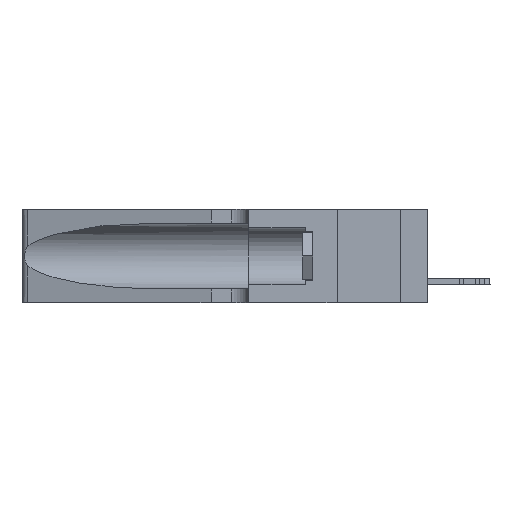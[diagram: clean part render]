
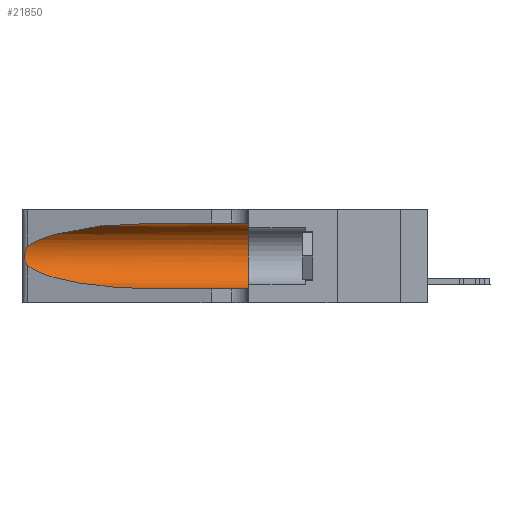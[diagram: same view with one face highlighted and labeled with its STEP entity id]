
A CAD part, left-side view. The second image highlights one B-rep face of the part: STEP entity #21850.
In plain terms, the highlighted cylindrical face has radius 3.308 mm (diameter 6.617 mm), a partial arc.
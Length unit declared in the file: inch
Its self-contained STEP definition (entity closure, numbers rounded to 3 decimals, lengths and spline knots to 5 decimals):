
#223 = FACE_OUTER_BOUND ( 'NONE', #41740, .T. ) ;
#475 = CARTESIAN_POINT ( 'NONE',  ( 0.1305, 0.35, 0.185 ) ) ;
#587 = VERTEX_POINT ( 'NONE', #12736 ) ;
#870 = ORIENTED_EDGE ( 'NONE', *, *, #23243, .T. ) ;
#1257 = CARTESIAN_POINT ( 'NONE',  ( 0.2373, 1.15595, 0.08982 ) ) ;
#1524 = ORIENTED_EDGE ( 'NONE', *, *, #5463, .F. ) ;
#1861 = CARTESIAN_POINT ( 'NONE',  ( 0.25639, 1.23184, 0.21858 ) ) ;
#2933 =( BOUNDED_CURVE ( )  B_SPLINE_CURVE ( 3, ( #22424, #42222, #25912, #22264 ),
 .UNSPECIFIED., .F., .F. ) 
 B_SPLINE_CURVE_WITH_KNOTS ( ( 4, 4 ),
 ( 1.5708, 2.84003 ),
 .UNSPECIFIED. ) 
 CURVE ( )  GEOMETRIC_REPRESENTATION_ITEM ( )  RATIONAL_B_SPLINE_CURVE ( ( 1., 0.87, 0.87, 1. ) ) 
 REPRESENTATION_ITEM ( '' )  );
#5463 = EDGE_CURVE ( 'NONE', #10100, #587, #26725, .T. ) ;
#5940 = DIRECTION ( 'NONE',  ( 0., -1., 0. ) ) ;
#6716 = VECTOR ( 'NONE', #9171, 39.37008 ) ;
#8279 = CIRCLE ( 'NONE', #35297, 0.13025 ) ;
#8772 = CARTESIAN_POINT ( 'NONE',  ( 0.26075, 1.23896, 0.19203 ) ) ;
#9171 = DIRECTION ( 'NONE',  ( 0., -1., 0. ) ) ;
#10028 = VERTEX_POINT ( 'NONE', #22106 ) ;
#10100 = VERTEX_POINT ( 'NONE', #35919 ) ;
#12147 = VERTEX_POINT ( 'NONE', #14419 ) ;
#12736 = CARTESIAN_POINT ( 'NONE',  ( 0.1305, 0.35, 0.31525 ) ) ;
#13600 = ORIENTED_EDGE ( 'NONE', *, *, #14310, .T. ) ;
#14310 = EDGE_CURVE ( 'NONE', #16075, #12147, #15464, .T. ) ;
#14419 = CARTESIAN_POINT ( 'NONE',  ( 0.1305, 0.35, 0.05475 ) ) ;
#14568 = CARTESIAN_POINT ( 'NONE',  ( 0.1305, 1.61858, 0.31525 ) ) ;
#15225 = CARTESIAN_POINT ( 'NONE',  ( 0.25555, 1.22994, 0.2215 ) ) ;
#15379 = CARTESIAN_POINT ( 'NONE',  ( 0.25787, 1.23484, 0.2124 ) ) ;
#15464 = LINE ( 'NONE', #30836, #6716 ) ;
#16075 = VERTEX_POINT ( 'NONE', #19417 ) ;
#17634 = CARTESIAN_POINT ( 'NONE',  ( 0.1305, 1.61858, 0.185 ) ) ;
#17783 = CARTESIAN_POINT ( 'NONE',  ( 0.1305, 0.72297, 0.05475 ) ) ;
#17888 = ORIENTED_EDGE ( 'NONE', *, *, #30081, .T. ) ;
#18008 = VECTOR ( 'NONE', #5940, 39.37008 ) ;
#19417 = CARTESIAN_POINT ( 'NONE',  ( 0.1305, 0.72297, 0.05475 ) ) ;
#21526 = CARTESIAN_POINT ( 'NONE',  ( 0.26075, 1.23896, 0.178 ) ) ;
#21850 = ADVANCED_FACE ( 'NONE', ( #223 ), #28533, .F. ) ;
#21956 = CARTESIAN_POINT ( 'NONE',  ( 0.25854, 1.2359, 0.20912 ) ) ;
#22106 = CARTESIAN_POINT ( 'NONE',  ( 0.25487, 1.22718, 0.14631 ) ) ;
#22264 = CARTESIAN_POINT ( 'NONE',  ( 0.25487, 1.22718, 0.22369 ) ) ;
#22424 = CARTESIAN_POINT ( 'NONE',  ( 0.1305, 0.72297, 0.31525 ) ) ;
#22768 = CARTESIAN_POINT ( 'NONE',  ( 0.25487, 1.22718, 0.22369 ) ) ;
#23243 = EDGE_CURVE ( 'NONE', #10100, #38508, #2933, .T. ) ;
#23575 = DIRECTION ( 'NONE',  ( 0., 1., 0. ) ) ;
#24788 = ORIENTED_EDGE ( 'NONE', *, *, #33444, .T. ) ;
#24831 = CARTESIAN_POINT ( 'NONE',  ( 0.26017, 1.23833, 0.17102 ) ) ;
#24858 = AXIS2_PLACEMENT_3D ( 'NONE', #17634, #40010, #40598 ) ;
#24983 = CARTESIAN_POINT ( 'NONE',  ( 0.25856, 1.23593, 0.16098 ) ) ;
#25912 = CARTESIAN_POINT ( 'NONE',  ( 0.2373, 1.15595, 0.28018 ) ) ;
#26725 = LINE ( 'NONE', #14568, #18008 ) ;
#26900 = DIRECTION ( 'NONE',  ( 0., 0., 1. ) ) ;
#27567 = CARTESIAN_POINT ( 'NONE',  ( 0.18966, 0.96281, 0.05475 ) ) ;
#28533 = CYLINDRICAL_SURFACE ( 'NONE', #24858, 0.13025 ) ;
#28671 =( BOUNDED_CURVE ( )  B_SPLINE_CURVE ( 3, ( #37457, #1257, #27567, #17783 ),
 .UNSPECIFIED., .F., .F. ) 
 B_SPLINE_CURVE_WITH_KNOTS ( ( 4, 4 ),
 ( 3.44316, 4.71239 ),
 .UNSPECIFIED. ) 
 CURVE ( )  GEOMETRIC_REPRESENTATION_ITEM ( )  RATIONAL_B_SPLINE_CURVE ( ( 1., 0.87, 0.87, 1. ) ) 
 REPRESENTATION_ITEM ( '' )  );
#30081 = EDGE_CURVE ( 'NONE', #38508, #10028, #34724, .T. ) ;
#30836 = CARTESIAN_POINT ( 'NONE',  ( 0.1305, 1.61858, 0.05475 ) ) ;
#32075 = EDGE_CURVE ( 'NONE', #587, #12147, #8279, .T. ) ;
#32460 = ORIENTED_EDGE ( 'NONE', *, *, #32075, .F. ) ;
#33444 = EDGE_CURVE ( 'NONE', #10028, #16075, #28671, .T. ) ;
#34724 = B_SPLINE_CURVE_WITH_KNOTS ( 'NONE', 3,
 ( #34758, #15225, #1861, #15379, #21956, #35047, #8772, #21526, #24831, #24983, #35193, #38188, #38333, #41762 ),
 .UNSPECIFIED., .F., .F.,
 ( 4, 2, 2, 2, 2, 2, 4 ),
 ( 0., 0.00027, 0.00053, 0.00107, 0.0016, 0.00187, 0.00214 ),
 .UNSPECIFIED. ) ;
#34758 = CARTESIAN_POINT ( 'NONE',  ( 0.25487, 1.22718, 0.22369 ) ) ;
#35047 = CARTESIAN_POINT ( 'NONE',  ( 0.26018, 1.23835, 0.19895 ) ) ;
#35193 = CARTESIAN_POINT ( 'NONE',  ( 0.25789, 1.23486, 0.15765 ) ) ;
#35297 = AXIS2_PLACEMENT_3D ( 'NONE', #475, #23575, #26900 ) ;
#35919 = CARTESIAN_POINT ( 'NONE',  ( 0.1305, 0.72297, 0.31525 ) ) ;
#37457 = CARTESIAN_POINT ( 'NONE',  ( 0.25487, 1.22718, 0.14631 ) ) ;
#38188 = CARTESIAN_POINT ( 'NONE',  ( 0.25639, 1.23186, 0.15144 ) ) ;
#38333 = CARTESIAN_POINT ( 'NONE',  ( 0.25555, 1.22993, 0.14849 ) ) ;
#38508 = VERTEX_POINT ( 'NONE', #22768 ) ;
#40010 = DIRECTION ( 'NONE',  ( 0., -1., 0. ) ) ;
#40598 = DIRECTION ( 'NONE',  ( 0., 0., -1. ) ) ;
#41740 = EDGE_LOOP ( 'NONE', ( #870, #17888, #24788, #13600, #32460, #1524 ) ) ;
#41762 = CARTESIAN_POINT ( 'NONE',  ( 0.25487, 1.22718, 0.14631 ) ) ;
#42222 = CARTESIAN_POINT ( 'NONE',  ( 0.18966, 0.96281, 0.31525 ) ) ;
